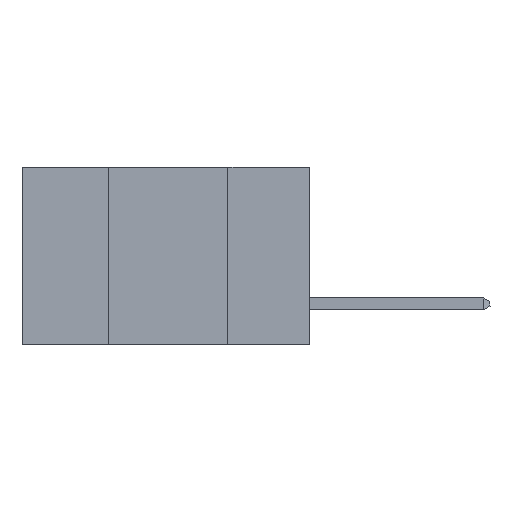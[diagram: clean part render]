
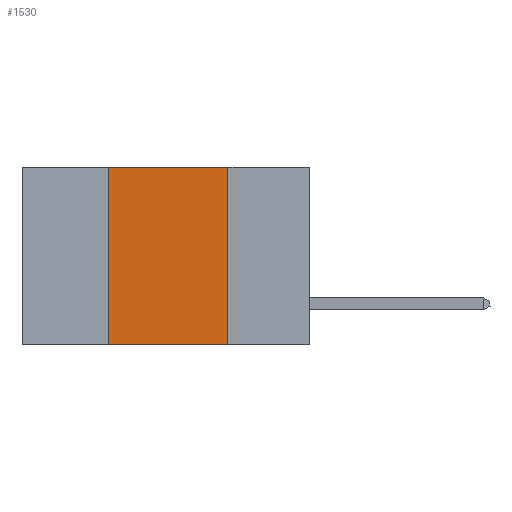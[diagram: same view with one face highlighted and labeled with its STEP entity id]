
A CAD part, left-side view. The second image highlights one B-rep face of the part: STEP entity #1530.
In plain terms, the highlighted planar face has unit normal (-1, 0, 0).
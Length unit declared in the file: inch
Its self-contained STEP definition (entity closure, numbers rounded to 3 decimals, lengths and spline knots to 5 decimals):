
#693 = ORIENTED_EDGE ( 'NONE', *, *, #10905, .F. ) ;
#805 = CARTESIAN_POINT ( 'NONE',  ( 0., 0.17, -0.37 ) ) ;
#1412 = CARTESIAN_POINT ( 'NONE',  ( 0., 0.42, -0.37 ) ) ;
#1530 = ADVANCED_FACE ( 'NONE', ( #4249 ), #5838, .F. ) ;
#1539 = VECTOR ( 'NONE', #20836, 39.37008 ) ;
#2006 = VECTOR ( 'NONE', #18142, 39.37008 ) ;
#2234 = LINE ( 'NONE', #19209, #19102 ) ;
#2436 = DIRECTION ( 'NONE',  ( 0., -1., 0. ) ) ;
#3028 = ORIENTED_EDGE ( 'NONE', *, *, #4210, .F. ) ;
#4210 = EDGE_CURVE ( 'NONE', #16462, #16545, #12792, .T. ) ;
#4249 = FACE_OUTER_BOUND ( 'NONE', #20540, .T. ) ;
#5838 = PLANE ( 'NONE',  #12810 ) ;
#6534 = LINE ( 'NONE', #9673, #2006 ) ;
#6909 = VERTEX_POINT ( 'NONE', #805 ) ;
#8430 = CARTESIAN_POINT ( 'NONE',  ( 0., 0.42, 0. ) ) ;
#9178 = DIRECTION ( 'NONE',  ( 0., 0., -1. ) ) ;
#9377 = CARTESIAN_POINT ( 'NONE',  ( 0., 0.42, 0. ) ) ;
#9673 = CARTESIAN_POINT ( 'NONE',  ( 0., 0.6, 0. ) ) ;
#10707 = ORIENTED_EDGE ( 'NONE', *, *, #14733, .T. ) ;
#10905 = EDGE_CURVE ( 'NONE', #14548, #6909, #18922, .T. ) ;
#10937 = ORIENTED_EDGE ( 'NONE', *, *, #21077, .F. ) ;
#12255 = VECTOR ( 'NONE', #21265, 39.37008 ) ;
#12792 = LINE ( 'NONE', #9377, #12255 ) ;
#12810 = AXIS2_PLACEMENT_3D ( 'NONE', #17570, #19265, #9178 ) ;
#14548 = VERTEX_POINT ( 'NONE', #20373 ) ;
#14733 = EDGE_CURVE ( 'NONE', #16462, #6909, #2234, .T. ) ;
#15888 = CARTESIAN_POINT ( 'NONE',  ( 0., 0.17, 0. ) ) ;
#16462 = VERTEX_POINT ( 'NONE', #1412 ) ;
#16545 = VERTEX_POINT ( 'NONE', #8430 ) ;
#17570 = CARTESIAN_POINT ( 'NONE',  ( 0., 0.6, 0. ) ) ;
#18142 = DIRECTION ( 'NONE',  ( 0., -1., 0. ) ) ;
#18922 = LINE ( 'NONE', #15888, #1539 ) ;
#19102 = VECTOR ( 'NONE', #2436, 39.37008 ) ;
#19209 = CARTESIAN_POINT ( 'NONE',  ( 0., 0.6, -0.37 ) ) ;
#19265 = DIRECTION ( 'NONE',  ( 1., 0., 0. ) ) ;
#20373 = CARTESIAN_POINT ( 'NONE',  ( 0., 0.17, 0. ) ) ;
#20540 = EDGE_LOOP ( 'NONE', ( #693, #10937, #3028, #10707 ) ) ;
#20836 = DIRECTION ( 'NONE',  ( 0., 0., -1. ) ) ;
#21077 = EDGE_CURVE ( 'NONE', #16545, #14548, #6534, .T. ) ;
#21265 = DIRECTION ( 'NONE',  ( 0., 0., 1. ) ) ;
